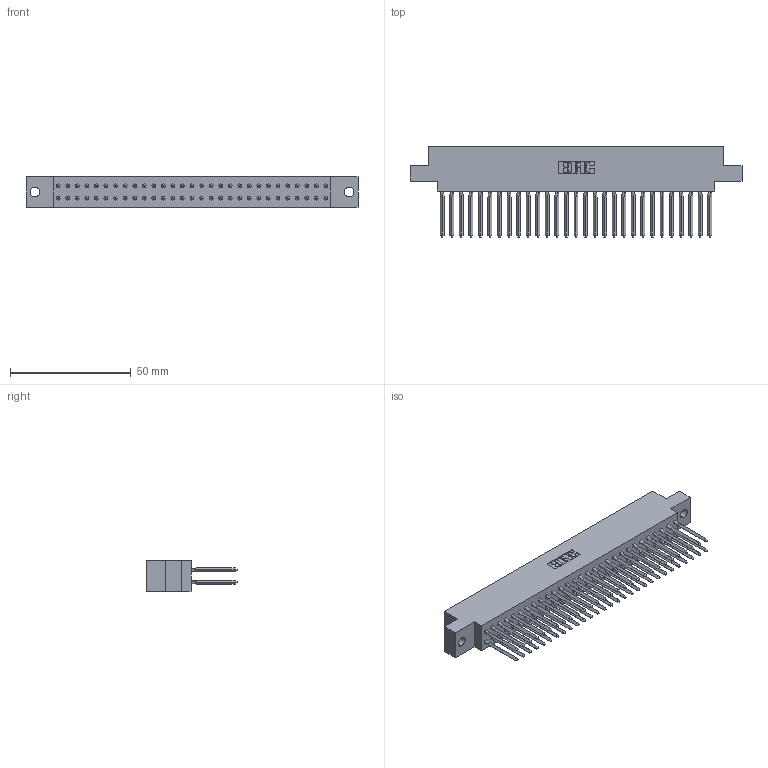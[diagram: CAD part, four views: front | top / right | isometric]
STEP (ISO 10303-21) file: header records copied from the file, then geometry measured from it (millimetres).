
FILE_DESCRIPTION (( 'STEP AP203' ), '1' );
FILE_NAME ('317-058-542-804.STEP', '2020-02-28T04:43:14', ( '' ), ( '' ), 'SwSTEP 2.0', 'SolidWorks 2016', '' );
FILE_SCHEMA (( 'CONFIG_CONTROL_DESIGN' ));
Length unit declared in the file: inch
Products named in the file (3): 317 Part_.156 Dia - TH; 317-290-003_542; 317-058-542-804
Assembly tree (59 placements, depth 2):
  317-058-542-804
    317 Part_.156 Dia - TH
    317-290-003_542  x58
Bounding box: 137.62 x 37.34 x 12.7 mm (x, y, z)
Volume: 22035.7 mm3; surface area: 30042.6 mm2
Topology: 59 solids, 59 shells, 3408 faces, 9555 edges, 6098 vertices
Faces by surface type: plane 2726, cylinder 450, bspline 232
Entity records: 42753 total; most frequent: CARTESIAN_POINT 7705, ORIENTED_EDGE 7368, DIRECTION 6220, EDGE_CURVE 3684, LINE 3514, VECTOR 3514, VERTEX_POINT 2450, AXIS2_PLACEMENT_3D 1353
